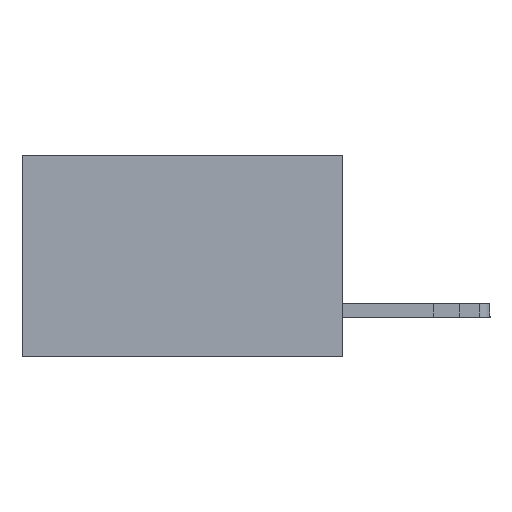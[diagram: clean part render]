
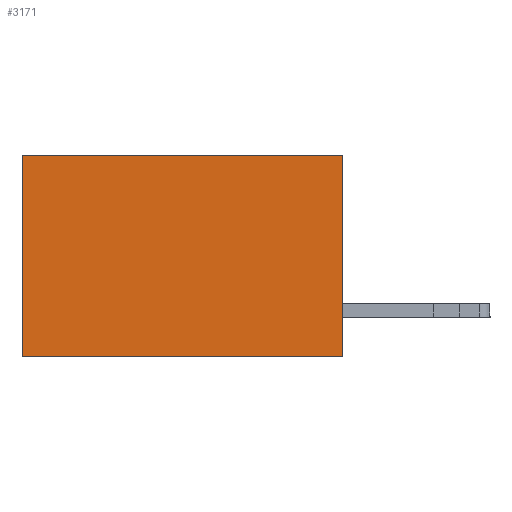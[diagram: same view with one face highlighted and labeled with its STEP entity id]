
A CAD part, left-side view. The second image highlights one B-rep face of the part: STEP entity #3171.
In plain terms, the highlighted planar face has unit normal (-1, 0, 0).
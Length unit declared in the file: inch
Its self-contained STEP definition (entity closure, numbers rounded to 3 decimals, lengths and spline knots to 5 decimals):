
#296 = VERTEX_POINT ( 'NONE', #4779 ) ;
#328 = VERTEX_POINT ( 'NONE', #15150 ) ;
#867 = DIRECTION ( 'NONE',  ( 0., 0., -1. ) ) ;
#1102 = AXIS2_PLACEMENT_3D ( 'NONE', #1373, #1137, #867 ) ;
#1137 = DIRECTION ( 'NONE',  ( 1., 0., 0. ) ) ;
#1373 = CARTESIAN_POINT ( 'NONE',  ( 0.277, 0., -0.37 ) ) ;
#1481 = PLANE ( 'NONE',  #1102 ) ;
#1542 = VERTEX_POINT ( 'NONE', #7759 ) ;
#2125 = LINE ( 'NONE', #11814, #5557 ) ;
#2194 = LINE ( 'NONE', #8779, #16515 ) ;
#3171 = ADVANCED_FACE ( 'NONE', ( #14622 ), #1481, .F. ) ;
#3397 = VECTOR ( 'NONE', #12548, 39.37008 ) ;
#4584 = EDGE_CURVE ( 'NONE', #1542, #328, #17593, .T. ) ;
#4779 = CARTESIAN_POINT ( 'NONE',  ( 0.277, 0., -0.37 ) ) ;
#5442 = CARTESIAN_POINT ( 'NONE',  ( 0.277, 0., -0.37 ) ) ;
#5557 = VECTOR ( 'NONE', #13184, 39.37008 ) ;
#6439 = ORIENTED_EDGE ( 'NONE', *, *, #8907, .F. ) ;
#6713 = ORIENTED_EDGE ( 'NONE', *, *, #14269, .T. ) ;
#7759 = CARTESIAN_POINT ( 'NONE',  ( 0.277, 0., 0. ) ) ;
#8466 = VECTOR ( 'NONE', #11036, 39.37008 ) ;
#8779 = CARTESIAN_POINT ( 'NONE',  ( 0.277, 0., -0.37 ) ) ;
#8907 = EDGE_CURVE ( 'NONE', #1542, #296, #15624, .T. ) ;
#9202 = CARTESIAN_POINT ( 'NONE',  ( 0.277, 0.59, -0.37 ) ) ;
#10642 = ORIENTED_EDGE ( 'NONE', *, *, #4584, .T. ) ;
#11036 = DIRECTION ( 'NONE',  ( 0., 0., -1. ) ) ;
#11081 = ORIENTED_EDGE ( 'NONE', *, *, #12619, .F. ) ;
#11543 = CARTESIAN_POINT ( 'NONE',  ( 0.277, 0., 0. ) ) ;
#11814 = CARTESIAN_POINT ( 'NONE',  ( 0.277, 0.59, -0.37 ) ) ;
#12548 = DIRECTION ( 'NONE',  ( 0., 1., 0. ) ) ;
#12619 = EDGE_CURVE ( 'NONE', #296, #17257, #2194, .T. ) ;
#13184 = DIRECTION ( 'NONE',  ( 0., 0., -1. ) ) ;
#14252 = DIRECTION ( 'NONE',  ( 0., 1., 0. ) ) ;
#14269 = EDGE_CURVE ( 'NONE', #328, #17257, #2125, .T. ) ;
#14622 = FACE_OUTER_BOUND ( 'NONE', #15755, .T. ) ;
#15150 = CARTESIAN_POINT ( 'NONE',  ( 0.277, 0.59, 0. ) ) ;
#15624 = LINE ( 'NONE', #5442, #8466 ) ;
#15755 = EDGE_LOOP ( 'NONE', ( #6713, #11081, #6439, #10642 ) ) ;
#16515 = VECTOR ( 'NONE', #14252, 39.37008 ) ;
#17257 = VERTEX_POINT ( 'NONE', #9202 ) ;
#17593 = LINE ( 'NONE', #11543, #3397 ) ;
